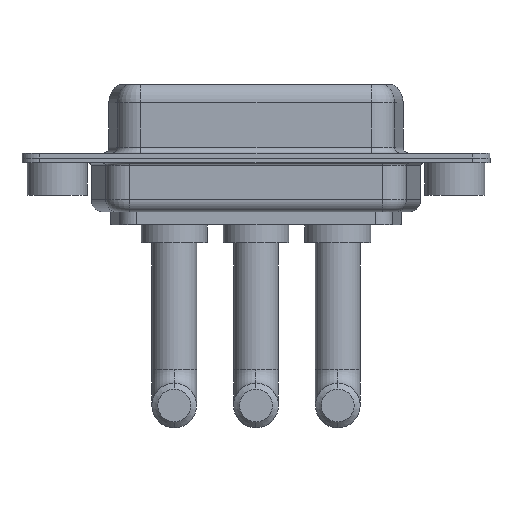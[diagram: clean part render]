
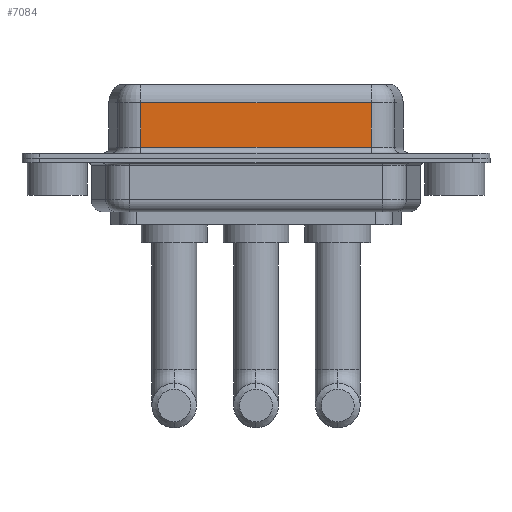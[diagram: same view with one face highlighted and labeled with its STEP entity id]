
A CAD part, front view. The second image highlights one B-rep face of the part: STEP entity #7084.
In plain terms, the highlighted planar face has unit normal (0, -1, 0).
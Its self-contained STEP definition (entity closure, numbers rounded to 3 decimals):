
#8 = VECTOR ( 'NONE', #11387, 1000. ) ;
#78 = CARTESIAN_POINT ( 'NONE',  ( 7.013, -3.95, 4.65 ) ) ;
#166 = CARTESIAN_POINT ( 'NONE',  ( 26.287, -3.95, 4.65 ) ) ;
#752 = VECTOR ( 'NONE', #1471, 1000. ) ;
#789 = LINE ( 'NONE', #7567, #8 ) ;
#1100 = ORIENTED_EDGE ( 'NONE', *, *, #2017, .T. ) ;
#1184 = VERTEX_POINT ( 'NONE', #8773 ) ;
#1471 = DIRECTION ( 'NONE',  ( 0., 0., -1. ) ) ;
#2017 = EDGE_CURVE ( 'NONE', #11702, #7592, #789, .T. ) ;
#3773 = PLANE ( 'NONE',  #10792 ) ;
#4493 = DIRECTION ( 'NONE',  ( 0., 0., -1. ) ) ;
#4749 = DIRECTION ( 'NONE',  ( 1., 0., 0. ) ) ;
#5220 = VECTOR ( 'NONE', #4749, 1000. ) ;
#5653 = EDGE_CURVE ( 'NONE', #7592, #7376, #6230, .T. ) ;
#6230 = LINE ( 'NONE', #10054, #752 ) ;
#6341 = CARTESIAN_POINT ( 'NONE',  ( 7.013, -3.95, 0.9 ) ) ;
#6665 = CARTESIAN_POINT ( 'NONE',  ( 26.287, -3.95, 0.9 ) ) ;
#6690 = CARTESIAN_POINT ( 'NONE',  ( 26.287, -3.95, 6.4 ) ) ;
#7084 = ADVANCED_FACE ( 'NONE', ( #8491 ), #3773, .F. ) ;
#7376 = VERTEX_POINT ( 'NONE', #6341 ) ;
#7567 = CARTESIAN_POINT ( 'NONE',  ( 26.287, -3.95, 4.65 ) ) ;
#7592 = VERTEX_POINT ( 'NONE', #78 ) ;
#7693 = EDGE_LOOP ( 'NONE', ( #11127, #1100, #9557, #8969 ) ) ;
#8491 = FACE_OUTER_BOUND ( 'NONE', #7693, .T. ) ;
#8766 = EDGE_CURVE ( 'NONE', #11702, #1184, #12149, .T. ) ;
#8773 = CARTESIAN_POINT ( 'NONE',  ( 26.287, -3.95, 0.9 ) ) ;
#8799 = VECTOR ( 'NONE', #4493, 1000. ) ;
#8969 = ORIENTED_EDGE ( 'NONE', *, *, #10828, .T. ) ;
#9557 = ORIENTED_EDGE ( 'NONE', *, *, #5653, .T. ) ;
#9594 = LINE ( 'NONE', #6665, #5220 ) ;
#9735 = DIRECTION ( 'NONE',  ( 0., 0., 1. ) ) ;
#10054 = CARTESIAN_POINT ( 'NONE',  ( 7.013, -3.95, 6.4 ) ) ;
#10613 = DIRECTION ( 'NONE',  ( 0., 1., 0. ) ) ;
#10792 = AXIS2_PLACEMENT_3D ( 'NONE', #6690, #10613, #9735 ) ;
#10828 = EDGE_CURVE ( 'NONE', #7376, #1184, #9594, .T. ) ;
#11127 = ORIENTED_EDGE ( 'NONE', *, *, #8766, .F. ) ;
#11387 = DIRECTION ( 'NONE',  ( -1., 0., 0. ) ) ;
#11702 = VERTEX_POINT ( 'NONE', #166 ) ;
#12027 = CARTESIAN_POINT ( 'NONE',  ( 26.287, -3.95, 6.4 ) ) ;
#12149 = LINE ( 'NONE', #12027, #8799 ) ;
